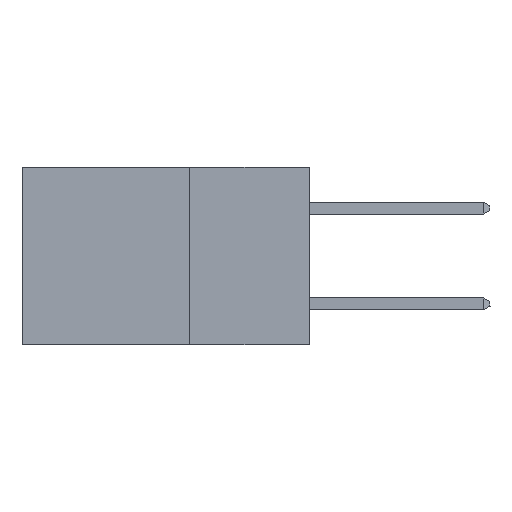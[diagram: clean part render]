
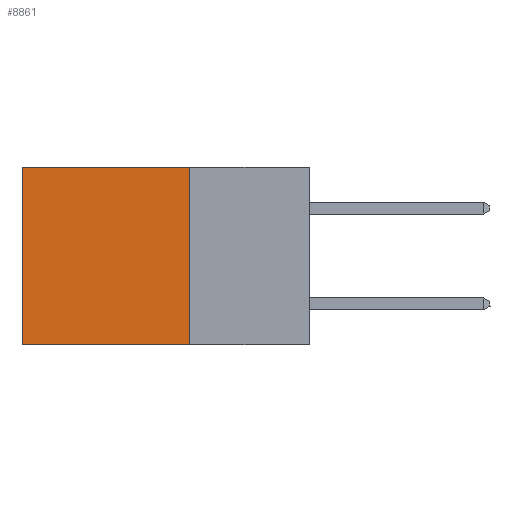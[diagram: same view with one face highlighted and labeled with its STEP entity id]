
A CAD part, left-side view. The second image highlights one B-rep face of the part: STEP entity #8861.
In plain terms, the highlighted planar face has unit normal (-1, 0, 0).
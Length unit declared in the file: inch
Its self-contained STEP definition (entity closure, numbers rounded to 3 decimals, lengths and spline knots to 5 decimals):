
#162 = CARTESIAN_POINT ( 'NONE',  ( 0.2875, 0.6, 0. ) ) ;
#242 = LINE ( 'NONE', #12442, #6717 ) ;
#1037 = ORIENTED_EDGE ( 'NONE', *, *, #5407, .T. ) ;
#1243 = PLANE ( 'NONE',  #13877 ) ;
#1294 = CARTESIAN_POINT ( 'NONE',  ( 0.2875, 0.25, 0. ) ) ;
#1525 = CARTESIAN_POINT ( 'NONE',  ( 0.2875, 0.25, 0. ) ) ;
#1535 = VECTOR ( 'NONE', #8570, 39.37008 ) ;
#2154 = EDGE_CURVE ( 'NONE', #14819, #6852, #3006, .T. ) ;
#2261 = VECTOR ( 'NONE', #9872, 39.37008 ) ;
#2507 = CARTESIAN_POINT ( 'NONE',  ( 0.2875, 0.6, -0.37 ) ) ;
#3006 = LINE ( 'NONE', #162, #1535 ) ;
#3187 = CARTESIAN_POINT ( 'NONE',  ( 0.2875, 0.25, -0.37 ) ) ;
#4873 = VERTEX_POINT ( 'NONE', #3187 ) ;
#5407 = EDGE_CURVE ( 'NONE', #13218, #14819, #8315, .T. ) ;
#6243 = CARTESIAN_POINT ( 'NONE',  ( 0.2875, 0.25, 0. ) ) ;
#6457 = VECTOR ( 'NONE', #12345, 39.37008 ) ;
#6717 = VECTOR ( 'NONE', #8976, 39.37008 ) ;
#6852 = VERTEX_POINT ( 'NONE', #2507 ) ;
#8315 = LINE ( 'NONE', #1525, #6457 ) ;
#8490 = FACE_OUTER_BOUND ( 'NONE', #12048, .T. ) ;
#8570 = DIRECTION ( 'NONE',  ( 0., 0., -1. ) ) ;
#8823 = ORIENTED_EDGE ( 'NONE', *, *, #11672, .F. ) ;
#8861 = ADVANCED_FACE ( 'NONE', ( #8490 ), #1243, .F. ) ;
#8976 = DIRECTION ( 'NONE',  ( 0., 1., 0. ) ) ;
#9332 = CARTESIAN_POINT ( 'NONE',  ( 0.2875, 0.6, 0. ) ) ;
#9872 = DIRECTION ( 'NONE',  ( 0., 0., -1. ) ) ;
#10773 = DIRECTION ( 'NONE',  ( 0., 0., -1. ) ) ;
#11007 = ORIENTED_EDGE ( 'NONE', *, *, #2154, .T. ) ;
#11672 = EDGE_CURVE ( 'NONE', #13218, #4873, #15379, .T. ) ;
#12048 = EDGE_LOOP ( 'NONE', ( #11007, #15211, #8823, #1037 ) ) ;
#12345 = DIRECTION ( 'NONE',  ( 0., 1., 0. ) ) ;
#12442 = CARTESIAN_POINT ( 'NONE',  ( 0.2875, 0.25, -0.37 ) ) ;
#12909 = EDGE_CURVE ( 'NONE', #4873, #6852, #242, .T. ) ;
#12985 = CARTESIAN_POINT ( 'NONE',  ( 0.2875, 0.25, 0. ) ) ;
#13152 = DIRECTION ( 'NONE',  ( 1., 0., 0. ) ) ;
#13218 = VERTEX_POINT ( 'NONE', #12985 ) ;
#13877 = AXIS2_PLACEMENT_3D ( 'NONE', #1294, #13152, #10773 ) ;
#14819 = VERTEX_POINT ( 'NONE', #9332 ) ;
#15211 = ORIENTED_EDGE ( 'NONE', *, *, #12909, .F. ) ;
#15379 = LINE ( 'NONE', #6243, #2261 ) ;
